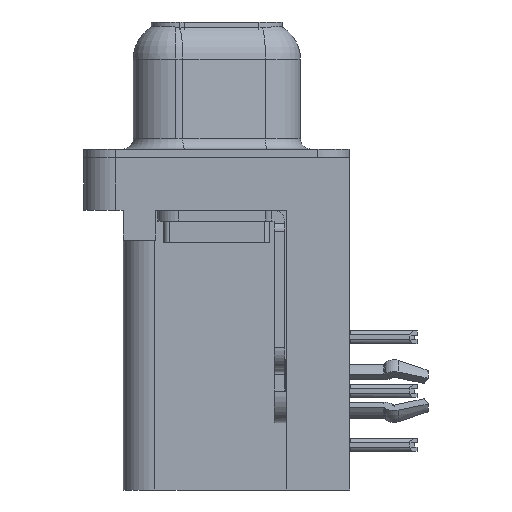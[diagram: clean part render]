
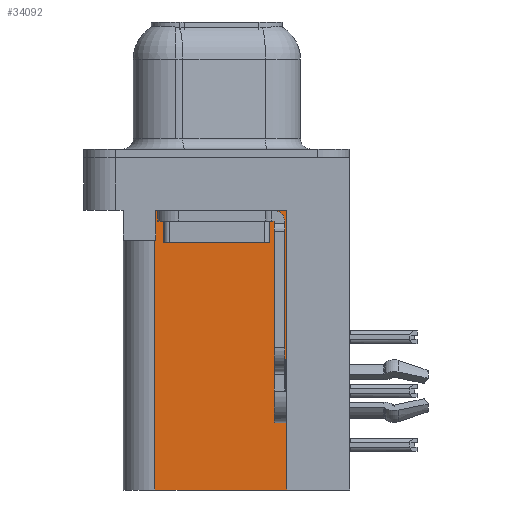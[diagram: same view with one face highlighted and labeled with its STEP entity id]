
A CAD part, left-side view. The second image highlights one B-rep face of the part: STEP entity #34092.
In plain terms, the highlighted planar face has unit normal (-1, 0, 0).
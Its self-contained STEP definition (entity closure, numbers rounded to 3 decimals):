
#76 = CARTESIAN_POINT ( 'NONE',  ( 3.765, -3.295, -15.7 ) ) ;
#1434 = CARTESIAN_POINT ( 'NONE',  ( 3.765, 2.895, -2.5 ) ) ;
#3123 = CARTESIAN_POINT ( 'NONE',  ( 3.765, -3.295, -15.7 ) ) ;
#3409 = AXIS2_PLACEMENT_3D ( 'NONE', #3123, #12217, #33100 ) ;
#3414 = CARTESIAN_POINT ( 'NONE',  ( 3.765, 2.925, -3.9 ) ) ;
#3900 = DIRECTION ( 'NONE',  ( 0., 1., 0. ) ) ;
#4203 = CARTESIAN_POINT ( 'NONE',  ( 3.765, -3.295, -2.5 ) ) ;
#4514 = VERTEX_POINT ( 'NONE', #3414 ) ;
#4901 = CARTESIAN_POINT ( 'NONE',  ( 3.765, 0., -3.9 ) ) ;
#6842 = VECTOR ( 'NONE', #10837, 1000. ) ;
#9215 = PLANE ( 'NONE',  #3409 ) ;
#9834 = CARTESIAN_POINT ( 'NONE',  ( 3.765, -3.295, -2.5 ) ) ;
#10837 = DIRECTION ( 'NONE',  ( 0., 0., -1. ) ) ;
#10849 = DIRECTION ( 'NONE',  ( 0., 0., 1. ) ) ;
#12217 = DIRECTION ( 'NONE',  ( 1., 0., 0. ) ) ;
#13257 = CARTESIAN_POINT ( 'NONE',  ( 3.765, 2.925, -15.7 ) ) ;
#13412 = VERTEX_POINT ( 'NONE', #28615 ) ;
#14380 = VERTEX_POINT ( 'NONE', #4203 ) ;
#14677 = ORIENTED_EDGE ( 'NONE', *, *, #22266, .T. ) ;
#15250 = VECTOR ( 'NONE', #37425, 1000. ) ;
#15849 = ORIENTED_EDGE ( 'NONE', *, *, #23760, .T. ) ;
#16539 = CARTESIAN_POINT ( 'NONE',  ( 3.765, -3.295, -15.7 ) ) ;
#17875 = ORIENTED_EDGE ( 'NONE', *, *, #22956, .T. ) ;
#18590 = VECTOR ( 'NONE', #3900, 1000. ) ;
#18987 = VECTOR ( 'NONE', #22819, 1000. ) ;
#20362 = LINE ( 'NONE', #31437, #30203 ) ;
#21044 = FACE_OUTER_BOUND ( 'NONE', #36743, .T. ) ;
#22266 = EDGE_CURVE ( 'NONE', #14380, #30215, #26552, .T. ) ;
#22563 = DIRECTION ( 'NONE',  ( 0., 0., 1. ) ) ;
#22594 = CARTESIAN_POINT ( 'NONE',  ( 3.765, 2.895, -3.9 ) ) ;
#22757 = LINE ( 'NONE', #37611, #30682 ) ;
#22819 = DIRECTION ( 'NONE',  ( 0., 1., 0. ) ) ;
#22956 = EDGE_CURVE ( 'NONE', #30215, #13412, #30692, .T. ) ;
#23760 = EDGE_CURVE ( 'NONE', #13412, #4514, #34870, .T. ) ;
#24200 = VERTEX_POINT ( 'NONE', #13257 ) ;
#26111 = ORIENTED_EDGE ( 'NONE', *, *, #26801, .F. ) ;
#26552 = LINE ( 'NONE', #9834, #18590 ) ;
#26801 = EDGE_CURVE ( 'NONE', #24200, #4514, #22757, .T. ) ;
#27263 = EDGE_CURVE ( 'NONE', #28177, #24200, #28340, .T. ) ;
#27315 = EDGE_CURVE ( 'NONE', #28177, #14380, #20362, .T. ) ;
#28177 = VERTEX_POINT ( 'NONE', #76 ) ;
#28340 = LINE ( 'NONE', #16539, #15250 ) ;
#28615 = CARTESIAN_POINT ( 'NONE',  ( 3.765, 2.895, -3.9 ) ) ;
#30203 = VECTOR ( 'NONE', #22563, 1000. ) ;
#30215 = VERTEX_POINT ( 'NONE', #1434 ) ;
#30520 = ORIENTED_EDGE ( 'NONE', *, *, #27315, .T. ) ;
#30682 = VECTOR ( 'NONE', #10849, 1000. ) ;
#30692 = LINE ( 'NONE', #22594, #6842 ) ;
#31437 = CARTESIAN_POINT ( 'NONE',  ( 3.765, -3.295, -15.7 ) ) ;
#33100 = DIRECTION ( 'NONE',  ( 0., 1., 0. ) ) ;
#34092 = ADVANCED_FACE ( 'NONE', ( #21044 ), #9215, .F. ) ;
#34870 = LINE ( 'NONE', #4901, #18987 ) ;
#35701 = ORIENTED_EDGE ( 'NONE', *, *, #27263, .F. ) ;
#36743 = EDGE_LOOP ( 'NONE', ( #14677, #17875, #15849, #26111, #35701, #30520 ) ) ;
#37425 = DIRECTION ( 'NONE',  ( 0., 1., 0. ) ) ;
#37611 = CARTESIAN_POINT ( 'NONE',  ( 3.765, 2.925, -15.7 ) ) ;
